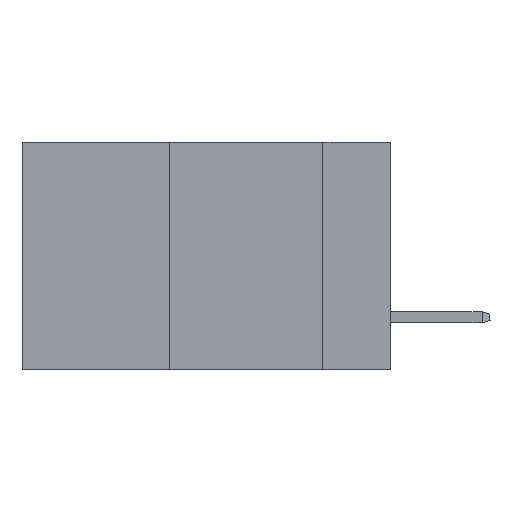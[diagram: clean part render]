
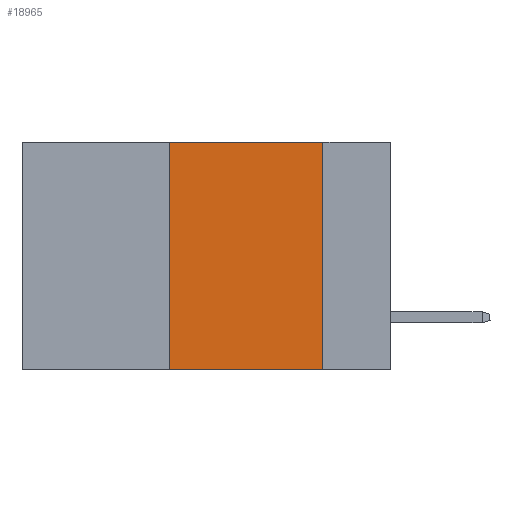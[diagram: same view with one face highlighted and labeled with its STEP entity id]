
A CAD part, left-side view. The second image highlights one B-rep face of the part: STEP entity #18965.
In plain terms, the highlighted planar face has unit normal (-1, 0, 0).
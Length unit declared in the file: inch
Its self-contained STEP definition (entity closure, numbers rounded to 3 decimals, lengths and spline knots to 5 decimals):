
#637 = LINE ( 'NONE', #6722, #12007 ) ;
#2498 = LINE ( 'NONE', #7032, #31864 ) ;
#3353 = PLANE ( 'NONE',  #49639 ) ;
#3847 = DIRECTION ( 'NONE',  ( 0., 0., 1. ) ) ;
#4313 = CARTESIAN_POINT ( 'NONE',  ( 0., 0.36, -0.37 ) ) ;
#6722 = CARTESIAN_POINT ( 'NONE',  ( 0., 0.11, 0. ) ) ;
#7010 = DIRECTION ( 'NONE',  ( 0., -1., 0. ) ) ;
#7032 = CARTESIAN_POINT ( 'NONE',  ( 0., 0.36, 0. ) ) ;
#7073 = ORIENTED_EDGE ( 'NONE', *, *, #19687, .F. ) ;
#7349 = DIRECTION ( 'NONE',  ( 1., 0., 0. ) ) ;
#8096 = EDGE_CURVE ( 'NONE', #25932, #16547, #637, .T. ) ;
#9019 = CARTESIAN_POINT ( 'NONE',  ( 0., 0.11, -0.37 ) ) ;
#10245 = VECTOR ( 'NONE', #42551, 39.37008 ) ;
#10835 = VERTEX_POINT ( 'NONE', #4313 ) ;
#11622 = CARTESIAN_POINT ( 'NONE',  ( 0., 0.6, 0. ) ) ;
#12007 = VECTOR ( 'NONE', #14567, 39.37008 ) ;
#14567 = DIRECTION ( 'NONE',  ( 0., 0., -1. ) ) ;
#15074 = CARTESIAN_POINT ( 'NONE',  ( 0., 0.6, -0.37 ) ) ;
#15417 = VECTOR ( 'NONE', #7010, 39.37008 ) ;
#16547 = VERTEX_POINT ( 'NONE', #9019 ) ;
#18572 = CARTESIAN_POINT ( 'NONE',  ( 0., 0.6, 0. ) ) ;
#18965 = ADVANCED_FACE ( 'NONE', ( #21258 ), #3353, .F. ) ;
#19222 = LINE ( 'NONE', #15074, #10245 ) ;
#19687 = EDGE_CURVE ( 'NONE', #41271, #25932, #37009, .T. ) ;
#20598 = ORIENTED_EDGE ( 'NONE', *, *, #8096, .F. ) ;
#21258 = FACE_OUTER_BOUND ( 'NONE', #24892, .T. ) ;
#23852 = EDGE_CURVE ( 'NONE', #10835, #16547, #19222, .T. ) ;
#23970 = CARTESIAN_POINT ( 'NONE',  ( 0., 0.11, 0. ) ) ;
#24892 = EDGE_LOOP ( 'NONE', ( #20598, #7073, #34243, #32295 ) ) ;
#25932 = VERTEX_POINT ( 'NONE', #23970 ) ;
#28774 = EDGE_CURVE ( 'NONE', #10835, #41271, #2498, .T. ) ;
#31864 = VECTOR ( 'NONE', #3847, 39.37008 ) ;
#32295 = ORIENTED_EDGE ( 'NONE', *, *, #23852, .T. ) ;
#34243 = ORIENTED_EDGE ( 'NONE', *, *, #28774, .F. ) ;
#35310 = CARTESIAN_POINT ( 'NONE',  ( 0., 0.36, 0. ) ) ;
#37009 = LINE ( 'NONE', #11622, #15417 ) ;
#41271 = VERTEX_POINT ( 'NONE', #35310 ) ;
#42551 = DIRECTION ( 'NONE',  ( 0., -1., 0. ) ) ;
#45416 = DIRECTION ( 'NONE',  ( 0., 0., -1. ) ) ;
#49639 = AXIS2_PLACEMENT_3D ( 'NONE', #18572, #7349, #45416 ) ;
